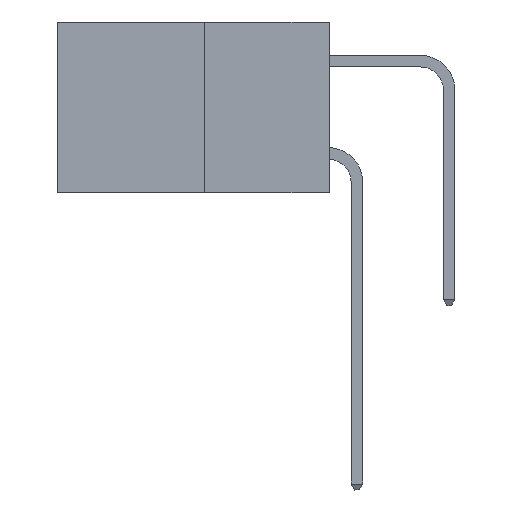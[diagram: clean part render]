
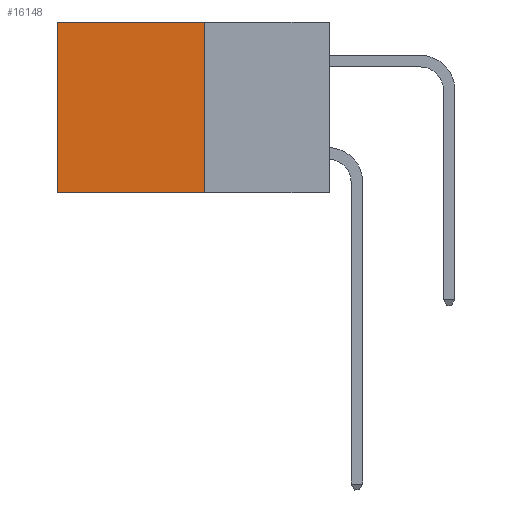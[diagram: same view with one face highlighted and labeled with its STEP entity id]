
A CAD part, left-side view. The second image highlights one B-rep face of the part: STEP entity #16148.
In plain terms, the highlighted planar face has unit normal (-1, 0, 0).
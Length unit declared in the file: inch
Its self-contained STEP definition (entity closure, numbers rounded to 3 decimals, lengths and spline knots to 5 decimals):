
#264 = VECTOR ( 'NONE', #14760, 39.37008 ) ;
#470 = LINE ( 'NONE', #4367, #7262 ) ;
#906 = ORIENTED_EDGE ( 'NONE', *, *, #16694, .T. ) ;
#1159 = CARTESIAN_POINT ( 'NONE',  ( 0.277, 0.27, -0.37 ) ) ;
#1656 = CARTESIAN_POINT ( 'NONE',  ( 0.277, 0.59, -0.37 ) ) ;
#2308 = AXIS2_PLACEMENT_3D ( 'NONE', #1159, #2528, #12040 ) ;
#2517 = CARTESIAN_POINT ( 'NONE',  ( 0.277, 0.27, 0. ) ) ;
#2528 = DIRECTION ( 'NONE',  ( 1., 0., 0. ) ) ;
#4241 = EDGE_LOOP ( 'NONE', ( #4500, #11279, #13643, #906 ) ) ;
#4367 = CARTESIAN_POINT ( 'NONE',  ( 0.277, 0.27, -0.37 ) ) ;
#4500 = ORIENTED_EDGE ( 'NONE', *, *, #12488, .T. ) ;
#4632 = VERTEX_POINT ( 'NONE', #13000 ) ;
#5797 = DIRECTION ( 'NONE',  ( 0., 0., -1. ) ) ;
#6048 = FACE_OUTER_BOUND ( 'NONE', #4241, .T. ) ;
#6924 = VERTEX_POINT ( 'NONE', #11707 ) ;
#7262 = VECTOR ( 'NONE', #5797, 39.37008 ) ;
#8807 = VECTOR ( 'NONE', #11205, 39.37008 ) ;
#9877 = CARTESIAN_POINT ( 'NONE',  ( 0.277, 0.27, -0.37 ) ) ;
#11097 = LINE ( 'NONE', #2517, #264 ) ;
#11205 = DIRECTION ( 'NONE',  ( 0., 1., 0. ) ) ;
#11279 = ORIENTED_EDGE ( 'NONE', *, *, #15738, .F. ) ;
#11707 = CARTESIAN_POINT ( 'NONE',  ( 0.277, 0.27, 0. ) ) ;
#11892 = VERTEX_POINT ( 'NONE', #14336 ) ;
#12040 = DIRECTION ( 'NONE',  ( 0., 0., -1. ) ) ;
#12488 = EDGE_CURVE ( 'NONE', #11892, #12728, #17211, .T. ) ;
#12728 = VERTEX_POINT ( 'NONE', #1656 ) ;
#13000 = CARTESIAN_POINT ( 'NONE',  ( 0.277, 0.27, -0.37 ) ) ;
#13643 = ORIENTED_EDGE ( 'NONE', *, *, #17314, .F. ) ;
#14336 = CARTESIAN_POINT ( 'NONE',  ( 0.277, 0.59, 0. ) ) ;
#14554 = CARTESIAN_POINT ( 'NONE',  ( 0.277, 0.59, -0.37 ) ) ;
#14760 = DIRECTION ( 'NONE',  ( 0., 1., 0. ) ) ;
#15738 = EDGE_CURVE ( 'NONE', #4632, #12728, #15993, .T. ) ;
#15887 = DIRECTION ( 'NONE',  ( 0., 0., -1. ) ) ;
#15993 = LINE ( 'NONE', #9877, #8807 ) ;
#16035 = PLANE ( 'NONE',  #2308 ) ;
#16148 = ADVANCED_FACE ( 'NONE', ( #6048 ), #16035, .F. ) ;
#16388 = VECTOR ( 'NONE', #15887, 39.37008 ) ;
#16694 = EDGE_CURVE ( 'NONE', #6924, #11892, #11097, .T. ) ;
#17211 = LINE ( 'NONE', #14554, #16388 ) ;
#17314 = EDGE_CURVE ( 'NONE', #6924, #4632, #470, .T. ) ;
